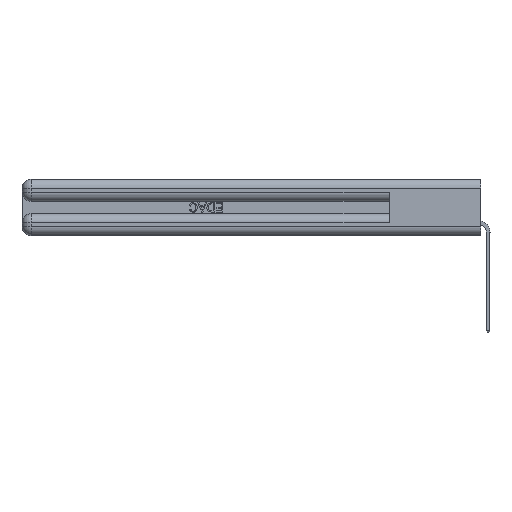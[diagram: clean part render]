
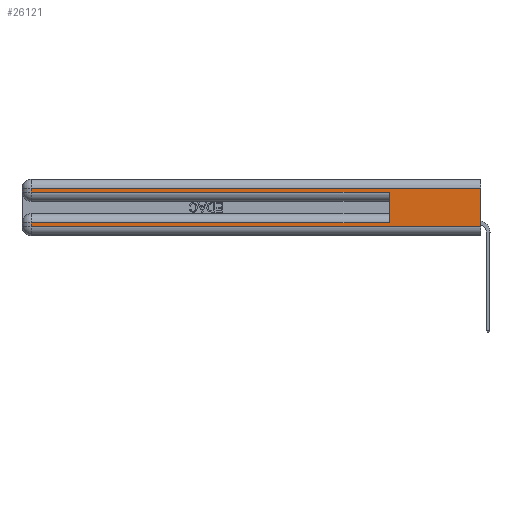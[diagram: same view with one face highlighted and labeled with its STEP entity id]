
A CAD part, left-side view. The second image highlights one B-rep face of the part: STEP entity #26121.
In plain terms, the highlighted planar face has unit normal (-1, 0, 0).
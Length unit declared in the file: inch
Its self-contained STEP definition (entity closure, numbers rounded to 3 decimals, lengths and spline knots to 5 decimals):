
#139 = ORIENTED_EDGE ( 'NONE', *, *, #2298, .T. ) ;
#363 = VECTOR ( 'NONE', #39635, 39.37008 ) ;
#1460 = VECTOR ( 'NONE', #1927, 39.37008 ) ;
#1771 = VERTEX_POINT ( 'NONE', #12581 ) ;
#1927 = DIRECTION ( 'NONE',  ( 0., -1., 0. ) ) ;
#2298 = EDGE_CURVE ( 'NONE', #40807, #3836, #15970, .T. ) ;
#2802 = VECTOR ( 'NONE', #10498, 39.37008 ) ;
#3095 = EDGE_CURVE ( 'NONE', #7397, #17623, #30009, .T. ) ;
#3836 = VERTEX_POINT ( 'NONE', #36542 ) ;
#4033 = ORIENTED_EDGE ( 'NONE', *, *, #8757, .T. ) ;
#4522 = LINE ( 'NONE', #14748, #1460 ) ;
#4748 = EDGE_CURVE ( 'NONE', #40807, #9535, #7620, .T. ) ;
#4921 = DIRECTION ( 'NONE',  ( 0., 0., -1. ) ) ;
#5681 = FACE_OUTER_BOUND ( 'NONE', #17815, .T. ) ;
#7336 = CARTESIAN_POINT ( 'NONE',  ( 0., 0., 0.37 ) ) ;
#7397 = VERTEX_POINT ( 'NONE', #34161 ) ;
#7620 = LINE ( 'NONE', #7893, #38456 ) ;
#7893 = CARTESIAN_POINT ( 'NONE',  ( 0., 0.6, 0.145 ) ) ;
#8625 = CARTESIAN_POINT ( 'NONE',  ( 0., 0., 0.06 ) ) ;
#8757 = EDGE_CURVE ( 'NONE', #38236, #1771, #12652, .T. ) ;
#9007 = DIRECTION ( 'NONE',  ( 0., 0., -1. ) ) ;
#9535 = VERTEX_POINT ( 'NONE', #14824 ) ;
#10498 = DIRECTION ( 'NONE',  ( 0., 1., 0. ) ) ;
#10815 = CARTESIAN_POINT ( 'NONE',  ( 0., 2.94, 0.37 ) ) ;
#11605 = ORIENTED_EDGE ( 'NONE', *, *, #25867, .T. ) ;
#12185 = VECTOR ( 'NONE', #27466, 39.37008 ) ;
#12230 = ORIENTED_EDGE ( 'NONE', *, *, #3095, .T. ) ;
#12581 = CARTESIAN_POINT ( 'NONE',  ( 0., 0., 0.06 ) ) ;
#12652 = LINE ( 'NONE', #8625, #12185 ) ;
#13360 = VECTOR ( 'NONE', #18208, 39.37008 ) ;
#14748 = CARTESIAN_POINT ( 'NONE',  ( 0., 0., 0.285 ) ) ;
#14824 = CARTESIAN_POINT ( 'NONE',  ( 0., 0.6, 0.285 ) ) ;
#15970 = LINE ( 'NONE', #23661, #13360 ) ;
#16547 = EDGE_CURVE ( 'NONE', #7397, #1771, #28625, .T. ) ;
#17623 = VERTEX_POINT ( 'NONE', #31151 ) ;
#17815 = EDGE_LOOP ( 'NONE', ( #29096, #12230, #25688, #11605, #21988, #139, #32039, #4033 ) ) ;
#18208 = DIRECTION ( 'NONE',  ( 0., 1., 0. ) ) ;
#19101 = EDGE_CURVE ( 'NONE', #3836, #38236, #40050, .T. ) ;
#19892 = CARTESIAN_POINT ( 'NONE',  ( 0., 2.94, 0.06 ) ) ;
#19950 = CARTESIAN_POINT ( 'NONE',  ( 0., 0.6, 0.085 ) ) ;
#21988 = ORIENTED_EDGE ( 'NONE', *, *, #4748, .F. ) ;
#22079 = VECTOR ( 'NONE', #39328, 39.37008 ) ;
#22667 = LINE ( 'NONE', #27099, #363 ) ;
#23661 = CARTESIAN_POINT ( 'NONE',  ( 0., 0., 0.085 ) ) ;
#24943 = VECTOR ( 'NONE', #4921, 39.37008 ) ;
#25332 = CARTESIAN_POINT ( 'NONE',  ( 0., 2.94, 0.285 ) ) ;
#25688 = ORIENTED_EDGE ( 'NONE', *, *, #39572, .T. ) ;
#25867 = EDGE_CURVE ( 'NONE', #38633, #9535, #4522, .T. ) ;
#26121 = ADVANCED_FACE ( 'NONE', ( #5681 ), #38430, .F. ) ;
#27099 = CARTESIAN_POINT ( 'NONE',  ( 0., 2.94, 0.37 ) ) ;
#27466 = DIRECTION ( 'NONE',  ( 0., -1., 0. ) ) ;
#28302 = DIRECTION ( 'NONE',  ( 1., 0., 0. ) ) ;
#28625 = LINE ( 'NONE', #7336, #22079 ) ;
#29096 = ORIENTED_EDGE ( 'NONE', *, *, #16547, .F. ) ;
#30009 = LINE ( 'NONE', #36430, #2802 ) ;
#30973 = AXIS2_PLACEMENT_3D ( 'NONE', #34909, #28302, #9007 ) ;
#31151 = CARTESIAN_POINT ( 'NONE',  ( 0., 2.94, 0.31 ) ) ;
#32039 = ORIENTED_EDGE ( 'NONE', *, *, #19101, .T. ) ;
#33823 = DIRECTION ( 'NONE',  ( 0., 0., 1. ) ) ;
#34161 = CARTESIAN_POINT ( 'NONE',  ( 0., 0., 0.31 ) ) ;
#34909 = CARTESIAN_POINT ( 'NONE',  ( 0., 0., 0.37 ) ) ;
#36430 = CARTESIAN_POINT ( 'NONE',  ( 0., 0., 0.31 ) ) ;
#36542 = CARTESIAN_POINT ( 'NONE',  ( 0., 2.94, 0.085 ) ) ;
#38236 = VERTEX_POINT ( 'NONE', #19892 ) ;
#38430 = PLANE ( 'NONE',  #30973 ) ;
#38456 = VECTOR ( 'NONE', #33823, 39.37008 ) ;
#38633 = VERTEX_POINT ( 'NONE', #25332 ) ;
#39328 = DIRECTION ( 'NONE',  ( 0., 0., -1. ) ) ;
#39572 = EDGE_CURVE ( 'NONE', #17623, #38633, #22667, .T. ) ;
#39635 = DIRECTION ( 'NONE',  ( 0., 0., -1. ) ) ;
#40050 = LINE ( 'NONE', #10815, #24943 ) ;
#40807 = VERTEX_POINT ( 'NONE', #19950 ) ;
